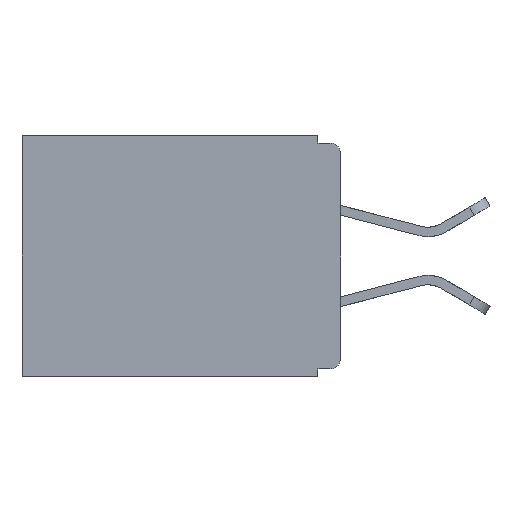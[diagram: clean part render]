
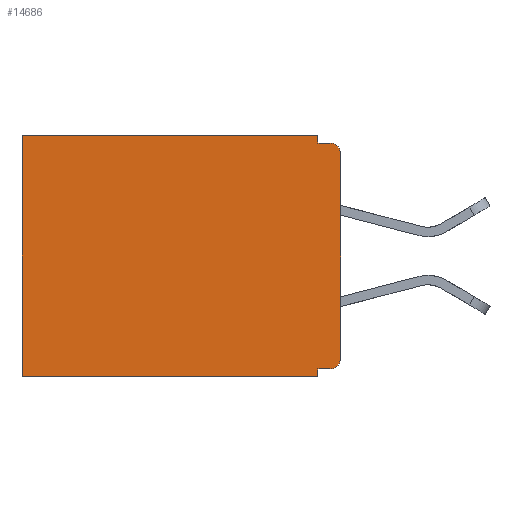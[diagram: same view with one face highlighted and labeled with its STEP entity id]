
A CAD part, left-side view. The second image highlights one B-rep face of the part: STEP entity #14686.
In plain terms, the highlighted planar face has unit normal (-1, 0, 0).
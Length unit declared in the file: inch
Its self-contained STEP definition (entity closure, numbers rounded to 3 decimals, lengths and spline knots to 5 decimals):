
#241 = AXIS2_PLACEMENT_3D ( 'NONE', #11326, #11236, #11213 ) ;
#280 = VERTEX_POINT ( 'NONE', #16008 ) ;
#410 = VERTEX_POINT ( 'NONE', #16953 ) ;
#428 = DIRECTION ( 'NONE',  ( 0., 0., -1. ) ) ;
#638 = ORIENTED_EDGE ( 'NONE', *, *, #6785, .T. ) ;
#2347 = CARTESIAN_POINT ( 'NONE',  ( 0.3, 0.015, -0.01 ) ) ;
#2614 = VERTEX_POINT ( 'NONE', #8191 ) ;
#2621 = PLANE ( 'NONE',  #18601 ) ;
#2646 = EDGE_CURVE ( 'NONE', #11692, #2614, #9352, .T. ) ;
#2766 = EDGE_CURVE ( 'NONE', #280, #3860, #14569, .T. ) ;
#2894 = CARTESIAN_POINT ( 'NONE',  ( 0.3, 0.031, 0. ) ) ;
#3231 = DIRECTION ( 'NONE',  ( 0., -1., 0. ) ) ;
#3337 = ORIENTED_EDGE ( 'NONE', *, *, #17929, .F. ) ;
#3604 = VERTEX_POINT ( 'NONE', #17161 ) ;
#3796 = EDGE_CURVE ( 'NONE', #12456, #410, #13691, .T. ) ;
#3860 = VERTEX_POINT ( 'NONE', #15932 ) ;
#3975 = FACE_OUTER_BOUND ( 'NONE', #16796, .T. ) ;
#4436 = VECTOR ( 'NONE', #11208, 39.37008 ) ;
#4698 = DIRECTION ( 'NONE',  ( 0., 0., -1. ) ) ;
#4721 = DIRECTION ( 'NONE',  ( -1., 0., 0. ) ) ;
#4880 = CARTESIAN_POINT ( 'NONE',  ( 0.3, 0.437, 0. ) ) ;
#5565 = VERTEX_POINT ( 'NONE', #4880 ) ;
#5657 = CARTESIAN_POINT ( 'NONE',  ( 0.3, 0., -0.33 ) ) ;
#5960 = VECTOR ( 'NONE', #15523, 39.37008 ) ;
#6200 = VECTOR ( 'NONE', #3231, 39.37008 ) ;
#6496 = EDGE_CURVE ( 'NONE', #5565, #7045, #8858, .T. ) ;
#6785 = EDGE_CURVE ( 'NONE', #3604, #8371, #7743, .T. ) ;
#6933 = VECTOR ( 'NONE', #12982, 39.37008 ) ;
#7045 = VERTEX_POINT ( 'NONE', #9779 ) ;
#7056 = CARTESIAN_POINT ( 'NONE',  ( 0.3, 0.015, -0.305 ) ) ;
#7101 = VECTOR ( 'NONE', #14609, 39.37008 ) ;
#7743 = CIRCLE ( 'NONE', #241, 0.015 ) ;
#8158 = DIRECTION ( 'NONE',  ( 0., 0., -1. ) ) ;
#8191 = CARTESIAN_POINT ( 'NONE',  ( 0.3, 0., -0.305 ) ) ;
#8201 = LINE ( 'NONE', #16411, #15160 ) ;
#8371 = VERTEX_POINT ( 'NONE', #2347 ) ;
#8675 = DIRECTION ( 'NONE',  ( 0., 0., -1. ) ) ;
#8699 = EDGE_CURVE ( 'NONE', #11692, #280, #12336, .T. ) ;
#8748 = ORIENTED_EDGE ( 'NONE', *, *, #10185, .T. ) ;
#8858 = LINE ( 'NONE', #11542, #4436 ) ;
#9352 = CIRCLE ( 'NONE', #12239, 0.015 ) ;
#9779 = CARTESIAN_POINT ( 'NONE',  ( 0.3, 0.437, -0.33 ) ) ;
#9804 = LINE ( 'NONE', #5657, #5960 ) ;
#9862 = CARTESIAN_POINT ( 'NONE',  ( 0.3, 0.015, -0.32 ) ) ;
#10185 = EDGE_CURVE ( 'NONE', #12456, #5565, #14828, .T. ) ;
#10564 = ORIENTED_EDGE ( 'NONE', *, *, #13543, .F. ) ;
#11208 = DIRECTION ( 'NONE',  ( 0., 0., -1. ) ) ;
#11213 = DIRECTION ( 'NONE',  ( 0., 0., -1. ) ) ;
#11236 = DIRECTION ( 'NONE',  ( -1., 0., 0. ) ) ;
#11326 = CARTESIAN_POINT ( 'NONE',  ( 0.3, 0.015, -0.025 ) ) ;
#11473 = ORIENTED_EDGE ( 'NONE', *, *, #2646, .T. ) ;
#11542 = CARTESIAN_POINT ( 'NONE',  ( 0.3, 0.437, -0.33 ) ) ;
#11692 = VERTEX_POINT ( 'NONE', #9862 ) ;
#11911 = VECTOR ( 'NONE', #15302, 39.37008 ) ;
#12239 = AXIS2_PLACEMENT_3D ( 'NONE', #7056, #4721, #4698 ) ;
#12336 = LINE ( 'NONE', #16829, #11911 ) ;
#12456 = VERTEX_POINT ( 'NONE', #2894 ) ;
#12619 = CARTESIAN_POINT ( 'NONE',  ( 0.3, 0.031, 0. ) ) ;
#12977 = CARTESIAN_POINT ( 'NONE',  ( 0.3, 0., 0. ) ) ;
#12980 = ORIENTED_EDGE ( 'NONE', *, *, #3796, .F. ) ;
#12982 = DIRECTION ( 'NONE',  ( 0., 1., 0. ) ) ;
#13543 = EDGE_CURVE ( 'NONE', #3860, #7045, #9804, .T. ) ;
#13691 = LINE ( 'NONE', #12619, #17277 ) ;
#13747 = LINE ( 'NONE', #16161, #6200 ) ;
#14259 = CARTESIAN_POINT ( 'NONE',  ( 0.3, 0., -0.33 ) ) ;
#14345 = EDGE_CURVE ( 'NONE', #410, #8371, #13747, .T. ) ;
#14569 = LINE ( 'NONE', #16112, #7101 ) ;
#14609 = DIRECTION ( 'NONE',  ( 0., 0., -1. ) ) ;
#14686 = ADVANCED_FACE ( 'NONE', ( #3975 ), #2621, .F. ) ;
#14828 = LINE ( 'NONE', #12977, #6933 ) ;
#15160 = VECTOR ( 'NONE', #428, 39.37008 ) ;
#15259 = ORIENTED_EDGE ( 'NONE', *, *, #14345, .F. ) ;
#15302 = DIRECTION ( 'NONE',  ( 0., 1., 0. ) ) ;
#15523 = DIRECTION ( 'NONE',  ( 0., 1., 0. ) ) ;
#15932 = CARTESIAN_POINT ( 'NONE',  ( 0.3, 0.031, -0.33 ) ) ;
#16008 = CARTESIAN_POINT ( 'NONE',  ( 0.3, 0.031, -0.32 ) ) ;
#16112 = CARTESIAN_POINT ( 'NONE',  ( 0.3, 0.031, -0.33 ) ) ;
#16161 = CARTESIAN_POINT ( 'NONE',  ( 0.3, 0., -0.01 ) ) ;
#16411 = CARTESIAN_POINT ( 'NONE',  ( 0.3, 0., -0.33 ) ) ;
#16564 = ORIENTED_EDGE ( 'NONE', *, *, #6496, .T. ) ;
#16796 = EDGE_LOOP ( 'NONE', ( #3337, #638, #15259, #12980, #8748, #16564, #10564, #17404, #17803, #11473 ) ) ;
#16829 = CARTESIAN_POINT ( 'NONE',  ( 0.3, 0., -0.32 ) ) ;
#16953 = CARTESIAN_POINT ( 'NONE',  ( 0.3, 0.031, -0.01 ) ) ;
#16969 = DIRECTION ( 'NONE',  ( 1., 0., 0. ) ) ;
#17161 = CARTESIAN_POINT ( 'NONE',  ( 0.3, 0., -0.025 ) ) ;
#17277 = VECTOR ( 'NONE', #8158, 39.37008 ) ;
#17404 = ORIENTED_EDGE ( 'NONE', *, *, #2766, .F. ) ;
#17803 = ORIENTED_EDGE ( 'NONE', *, *, #8699, .F. ) ;
#17929 = EDGE_CURVE ( 'NONE', #3604, #2614, #8201, .T. ) ;
#18601 = AXIS2_PLACEMENT_3D ( 'NONE', #14259, #16969, #8675 ) ;
